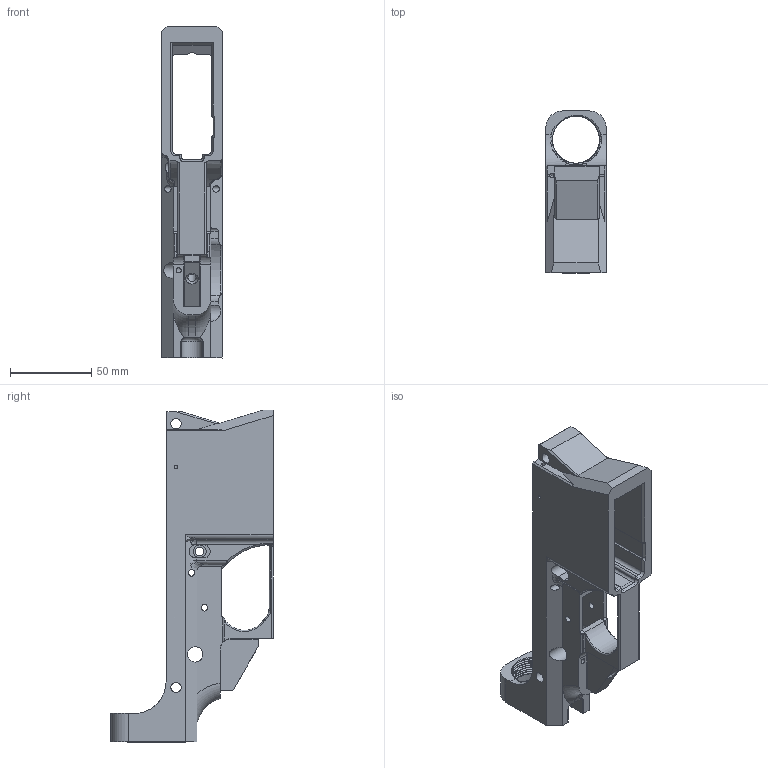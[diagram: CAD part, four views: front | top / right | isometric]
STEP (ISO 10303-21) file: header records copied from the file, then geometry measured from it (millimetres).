
FILE_DESCRIPTION(/* description */ (''),/* implementation_level */ '2;1');
FILE_NAME(/* name */ 'Vanguard - Fixed Dimensions V1.7.stp',/* time_stamp */ '2020-04-28T12:21:44-05:00',/* author */ ('johne'),/* organization */ (''),/* preprocessor_version */ 'ST-DEVELOPER v18',/* originating_system */ 'Autodesk Inventor 2020',/* authorisation */ '');
FILE_SCHEMA (('AUTOMOTIVE_DESIGN { 1 0 10303 214 3 1 1 }'));
Length unit declared in the file: inch
Products named in the file (1): Vanguard - Fixed Dimensions V1.7
Bounding box: 37.13 x 99.69 x 203.77 mm (x, y, z)
Volume: 175904.1 mm3; surface area: 62721 mm2
Topology: 1 solids, 1 shells, 482 faces, 1396 edges, 905 vertices
Faces by surface type: cylinder 165, plane 138, bspline 127, torus 30, cone 18, sphere 4
Full cylindrical faces by diameter (mm): 1.981 x1, 2.362 x1, 2.464 x1, 3.175 x1, 3.969 x5, 5.105 x1, 5.182 x1, 6.35 x4, 6.477 x1, 6.858 x1, 7.938 x1, 9.55 x2, 28.848 x6, 31.302 x1
Entity records: 27302 total; most frequent: CARTESIAN_POINT 15405, ORIENTED_EDGE 2784, DIRECTION 2084, EDGE_CURVE 1392, VERTEX_POINT 905, AXIS2_PLACEMENT_3D 757, LINE 570, VECTOR 570
